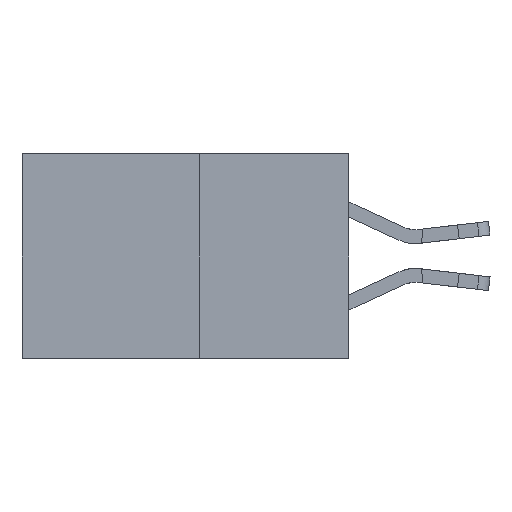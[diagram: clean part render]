
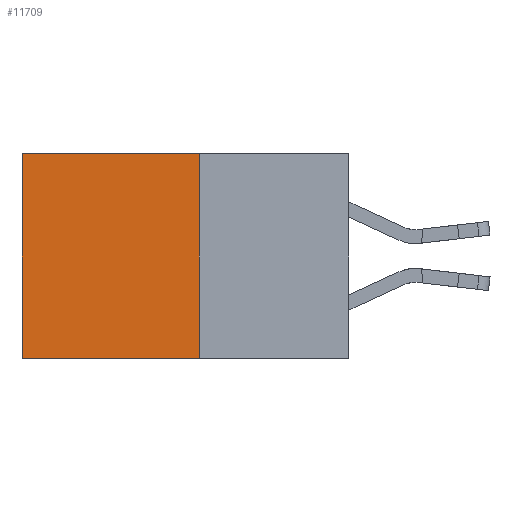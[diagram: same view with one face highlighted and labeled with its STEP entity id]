
A CAD part, left-side view. The second image highlights one B-rep face of the part: STEP entity #11709.
In plain terms, the highlighted planar face has unit normal (-1, 0, 0).
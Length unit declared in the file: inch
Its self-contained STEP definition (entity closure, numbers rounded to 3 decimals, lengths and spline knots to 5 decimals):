
#975 = CARTESIAN_POINT ( 'NONE',  ( 0.277, 0.27, -0.37 ) ) ;
#1963 = ORIENTED_EDGE ( 'NONE', *, *, #21120, .F. ) ;
#2887 = VERTEX_POINT ( 'NONE', #2911 ) ;
#2911 = CARTESIAN_POINT ( 'NONE',  ( 0.277, 0.27, -0.37 ) ) ;
#3108 = CARTESIAN_POINT ( 'NONE',  ( 0.277, 0.27, 0. ) ) ;
#3340 = EDGE_CURVE ( 'NONE', #11690, #3844, #15044, .T. ) ;
#3826 = CARTESIAN_POINT ( 'NONE',  ( 0.277, 0.27, -0.37 ) ) ;
#3844 = VERTEX_POINT ( 'NONE', #18725 ) ;
#4453 = DIRECTION ( 'NONE',  ( 0., 0., -1. ) ) ;
#5749 = VECTOR ( 'NONE', #17650, 39.37008 ) ;
#5757 = CARTESIAN_POINT ( 'NONE',  ( 0.277, 0.27, 0. ) ) ;
#5864 = LINE ( 'NONE', #3108, #10801 ) ;
#7523 = LINE ( 'NONE', #14089, #16704 ) ;
#8975 = LINE ( 'NONE', #3826, #17608 ) ;
#9875 = ORIENTED_EDGE ( 'NONE', *, *, #3340, .T. ) ;
#9913 = ORIENTED_EDGE ( 'NONE', *, *, #20816, .T. ) ;
#10648 = FACE_OUTER_BOUND ( 'NONE', #18415, .T. ) ;
#10801 = VECTOR ( 'NONE', #16285, 39.37008 ) ;
#11084 = PLANE ( 'NONE',  #16116 ) ;
#11437 = ORIENTED_EDGE ( 'NONE', *, *, #12276, .F. ) ;
#11690 = VERTEX_POINT ( 'NONE', #12661 ) ;
#11709 = ADVANCED_FACE ( 'NONE', ( #10648 ), #11084, .F. ) ;
#12276 = EDGE_CURVE ( 'NONE', #17906, #2887, #7523, .T. ) ;
#12661 = CARTESIAN_POINT ( 'NONE',  ( 0.277, 0.59, 0. ) ) ;
#13793 = DIRECTION ( 'NONE',  ( 0., 1., 0. ) ) ;
#14089 = CARTESIAN_POINT ( 'NONE',  ( 0.277, 0.27, -0.37 ) ) ;
#14395 = DIRECTION ( 'NONE',  ( 1., 0., 0. ) ) ;
#15044 = LINE ( 'NONE', #17680, #5749 ) ;
#15667 = DIRECTION ( 'NONE',  ( 0., 0., -1. ) ) ;
#16116 = AXIS2_PLACEMENT_3D ( 'NONE', #975, #14395, #4453 ) ;
#16285 = DIRECTION ( 'NONE',  ( 0., 1., 0. ) ) ;
#16704 = VECTOR ( 'NONE', #15667, 39.37008 ) ;
#17608 = VECTOR ( 'NONE', #13793, 39.37008 ) ;
#17650 = DIRECTION ( 'NONE',  ( 0., 0., -1. ) ) ;
#17680 = CARTESIAN_POINT ( 'NONE',  ( 0.277, 0.59, -0.37 ) ) ;
#17906 = VERTEX_POINT ( 'NONE', #5757 ) ;
#18415 = EDGE_LOOP ( 'NONE', ( #9875, #1963, #11437, #9913 ) ) ;
#18725 = CARTESIAN_POINT ( 'NONE',  ( 0.277, 0.59, -0.37 ) ) ;
#20816 = EDGE_CURVE ( 'NONE', #17906, #11690, #5864, .T. ) ;
#21120 = EDGE_CURVE ( 'NONE', #2887, #3844, #8975, .T. ) ;
